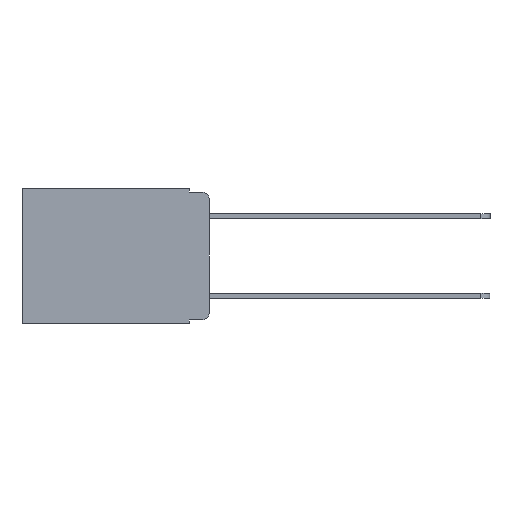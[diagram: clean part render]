
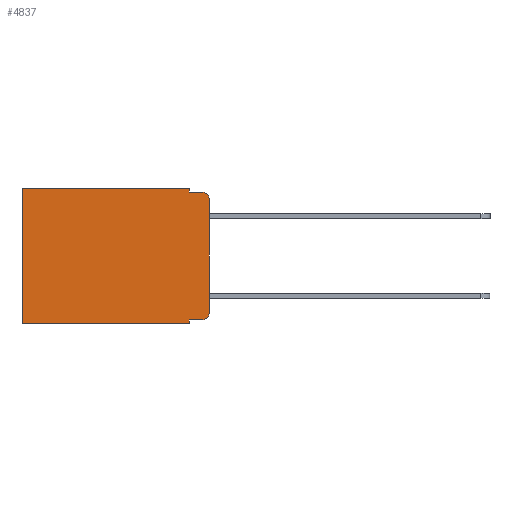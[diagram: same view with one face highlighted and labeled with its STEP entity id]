
A CAD part, left-side view. The second image highlights one B-rep face of the part: STEP entity #4837.
In plain terms, the highlighted planar face has unit normal (-1, 0, 0).
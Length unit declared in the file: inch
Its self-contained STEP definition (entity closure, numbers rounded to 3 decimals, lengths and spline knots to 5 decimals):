
#87 = VERTEX_POINT ( 'NONE', #6429 ) ;
#117 = VECTOR ( 'NONE', #5206, 39.37008 ) ;
#153 = CARTESIAN_POINT ( 'NONE',  ( 0.298, 0., -0.313 ) ) ;
#303 = VERTEX_POINT ( 'NONE', #1823 ) ;
#394 = VECTOR ( 'NONE', #6381, 39.37008 ) ;
#427 = DIRECTION ( 'NONE',  ( -1., 0., 0. ) ) ;
#780 = DIRECTION ( 'NONE',  ( 0., 0., -1. ) ) ;
#924 = CARTESIAN_POINT ( 'NONE',  ( 0.298, 0.02, -0.313 ) ) ;
#946 = DIRECTION ( 'NONE',  ( -1., 0., 0. ) ) ;
#1218 = EDGE_CURVE ( 'NONE', #7965, #7948, #1227, .T. ) ;
#1227 = LINE ( 'NONE', #5752, #8379 ) ;
#1460 = DIRECTION ( 'NONE',  ( 0., 0., -1. ) ) ;
#1612 = LINE ( 'NONE', #7736, #8652 ) ;
#1730 = LINE ( 'NONE', #2710, #5611 ) ;
#1748 = CIRCLE ( 'NONE', #5927, 0.02 ) ;
#1803 = EDGE_CURVE ( 'NONE', #2533, #2404, #1748, .T. ) ;
#1823 = CARTESIAN_POINT ( 'NONE',  ( 0.298, 0.051, 0. ) ) ;
#1853 = DIRECTION ( 'NONE',  ( 0., 0., -1. ) ) ;
#1866 = ORIENTED_EDGE ( 'NONE', *, *, #4588, .F. ) ;
#1867 = EDGE_CURVE ( 'NONE', #4569, #3611, #3335, .T. ) ;
#1890 = ORIENTED_EDGE ( 'NONE', *, *, #7601, .F. ) ;
#1980 = PLANE ( 'NONE',  #5184 ) ;
#2155 = VERTEX_POINT ( 'NONE', #3262 ) ;
#2181 = ORIENTED_EDGE ( 'NONE', *, *, #1867, .T. ) ;
#2297 = EDGE_CURVE ( 'NONE', #87, #2337, #6574, .T. ) ;
#2337 = VERTEX_POINT ( 'NONE', #7412 ) ;
#2341 = LINE ( 'NONE', #5586, #5719 ) ;
#2344 = ORIENTED_EDGE ( 'NONE', *, *, #5234, .T. ) ;
#2404 = VERTEX_POINT ( 'NONE', #153 ) ;
#2442 = ORIENTED_EDGE ( 'NONE', *, *, #2910, .F. ) ;
#2533 = VERTEX_POINT ( 'NONE', #7658 ) ;
#2575 = LINE ( 'NONE', #7749, #394 ) ;
#2662 = ORIENTED_EDGE ( 'NONE', *, *, #4765, .F. ) ;
#2679 = CARTESIAN_POINT ( 'NONE',  ( 0.298, 0.02, -0.03 ) ) ;
#2710 = CARTESIAN_POINT ( 'NONE',  ( 0.298, 0., 0. ) ) ;
#2830 = ORIENTED_EDGE ( 'NONE', *, *, #1218, .T. ) ;
#2834 = EDGE_CURVE ( 'NONE', #87, #2533, #2341, .T. ) ;
#2910 = EDGE_CURVE ( 'NONE', #303, #2155, #1612, .T. ) ;
#2931 = ORIENTED_EDGE ( 'NONE', *, *, #2834, .T. ) ;
#2992 = ORIENTED_EDGE ( 'NONE', *, *, #2297, .F. ) ;
#2998 = CARTESIAN_POINT ( 'NONE',  ( 0.298, 0., 0. ) ) ;
#3058 = DIRECTION ( 'NONE',  ( 0., 0., -1. ) ) ;
#3082 = ORIENTED_EDGE ( 'NONE', *, *, #1803, .T. ) ;
#3262 = CARTESIAN_POINT ( 'NONE',  ( 0.298, 0.051, -0.01 ) ) ;
#3335 = CIRCLE ( 'NONE', #6760, 0.02 ) ;
#3604 = EDGE_LOOP ( 'NONE', ( #1866, #2181, #1890, #2442, #2344, #2830, #2662, #2992, #2931, #3082 ) ) ;
#3611 = VERTEX_POINT ( 'NONE', #4082 ) ;
#3618 = DIRECTION ( 'NONE',  ( 1., 0., 0. ) ) ;
#4082 = CARTESIAN_POINT ( 'NONE',  ( 0.298, 0.02, -0.01 ) ) ;
#4569 = VERTEX_POINT ( 'NONE', #5393 ) ;
#4588 = EDGE_CURVE ( 'NONE', #4569, #2404, #6023, .T. ) ;
#4765 = EDGE_CURVE ( 'NONE', #2337, #7948, #9050, .T. ) ;
#4837 = ADVANCED_FACE ( 'NONE', ( #7027 ), #1980, .F. ) ;
#5171 = CARTESIAN_POINT ( 'NONE',  ( 0.298, 0.473, -0.343 ) ) ;
#5184 = AXIS2_PLACEMENT_3D ( 'NONE', #7557, #3618, #7248 ) ;
#5206 = DIRECTION ( 'NONE',  ( 0., 1., 0. ) ) ;
#5234 = EDGE_CURVE ( 'NONE', #303, #7965, #1730, .T. ) ;
#5393 = CARTESIAN_POINT ( 'NONE',  ( 0.298, 0., -0.03 ) ) ;
#5438 = CARTESIAN_POINT ( 'NONE',  ( 0.298, 0., -0.343 ) ) ;
#5586 = CARTESIAN_POINT ( 'NONE',  ( 0.298, 0.051, -0.333 ) ) ;
#5611 = VECTOR ( 'NONE', #7333, 39.37008 ) ;
#5719 = VECTOR ( 'NONE', #7472, 39.37008 ) ;
#5752 = CARTESIAN_POINT ( 'NONE',  ( 0.298, 0.473, 0. ) ) ;
#5927 = AXIS2_PLACEMENT_3D ( 'NONE', #924, #946, #3058 ) ;
#6023 = LINE ( 'NONE', #2998, #6588 ) ;
#6381 = DIRECTION ( 'NONE',  ( 0., -1., 0. ) ) ;
#6384 = CARTESIAN_POINT ( 'NONE',  ( 0.298, 0.473, 0. ) ) ;
#6421 = DIRECTION ( 'NONE',  ( 0., 0., -1. ) ) ;
#6429 = CARTESIAN_POINT ( 'NONE',  ( 0.298, 0.051, -0.333 ) ) ;
#6432 = CARTESIAN_POINT ( 'NONE',  ( 0.298, 0.051, 0. ) ) ;
#6574 = LINE ( 'NONE', #6432, #9044 ) ;
#6588 = VECTOR ( 'NONE', #1853, 39.37008 ) ;
#6760 = AXIS2_PLACEMENT_3D ( 'NONE', #2679, #427, #8394 ) ;
#7027 = FACE_OUTER_BOUND ( 'NONE', #3604, .T. ) ;
#7248 = DIRECTION ( 'NONE',  ( 0., 0., -1. ) ) ;
#7333 = DIRECTION ( 'NONE',  ( 0., 1., 0. ) ) ;
#7412 = CARTESIAN_POINT ( 'NONE',  ( 0.298, 0.051, -0.343 ) ) ;
#7472 = DIRECTION ( 'NONE',  ( 0., -1., 0. ) ) ;
#7557 = CARTESIAN_POINT ( 'NONE',  ( 0.298, 0., 0. ) ) ;
#7601 = EDGE_CURVE ( 'NONE', #2155, #3611, #2575, .T. ) ;
#7658 = CARTESIAN_POINT ( 'NONE',  ( 0.298, 0.02, -0.333 ) ) ;
#7736 = CARTESIAN_POINT ( 'NONE',  ( 0.298, 0.051, 0. ) ) ;
#7749 = CARTESIAN_POINT ( 'NONE',  ( 0.298, 0.051, -0.01 ) ) ;
#7948 = VERTEX_POINT ( 'NONE', #5171 ) ;
#7965 = VERTEX_POINT ( 'NONE', #6384 ) ;
#8379 = VECTOR ( 'NONE', #1460, 39.37008 ) ;
#8394 = DIRECTION ( 'NONE',  ( 0., 0., -1. ) ) ;
#8652 = VECTOR ( 'NONE', #780, 39.37008 ) ;
#9044 = VECTOR ( 'NONE', #6421, 39.37008 ) ;
#9050 = LINE ( 'NONE', #5438, #117 ) ;
